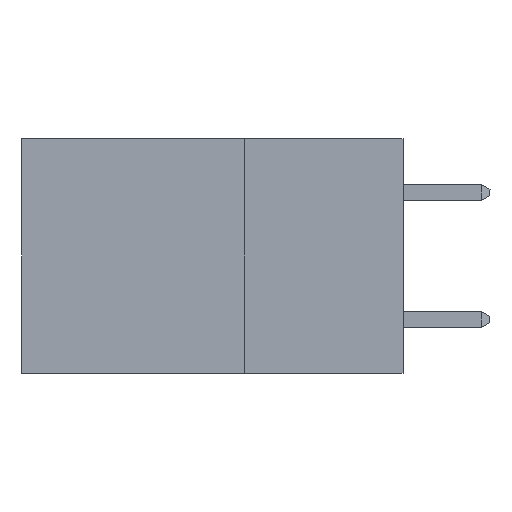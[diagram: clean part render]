
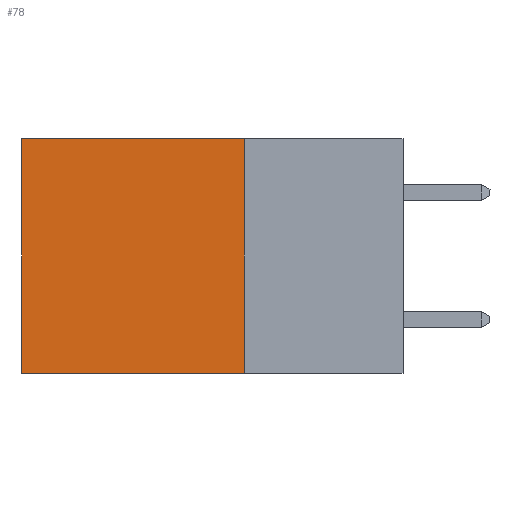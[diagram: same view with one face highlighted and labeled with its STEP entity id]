
A CAD part, left-side view. The second image highlights one B-rep face of the part: STEP entity #78.
In plain terms, the highlighted planar face has unit normal (-1, 0, 0).
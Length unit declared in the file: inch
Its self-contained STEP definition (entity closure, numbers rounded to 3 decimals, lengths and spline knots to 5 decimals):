
#54 = CARTESIAN_POINT ( 'NONE',  ( 0.2875, 0.25, 0. ) ) ;
#78 = ADVANCED_FACE ( 'NONE', ( #9329 ), #5982, .F. ) ;
#121 = DIRECTION ( 'NONE',  ( 0., 0., -1. ) ) ;
#945 = EDGE_CURVE ( 'NONE', #6502, #9573, #3906, .T. ) ;
#1660 = VERTEX_POINT ( 'NONE', #6087 ) ;
#1894 = DIRECTION ( 'NONE',  ( 0., 0., -1. ) ) ;
#2031 = CARTESIAN_POINT ( 'NONE',  ( 0.2875, 0.25, 0. ) ) ;
#2287 = EDGE_CURVE ( 'NONE', #6502, #1660, #8548, .T. ) ;
#2436 = DIRECTION ( 'NONE',  ( 1., 0., 0. ) ) ;
#2835 = DIRECTION ( 'NONE',  ( 0., 1., 0. ) ) ;
#3402 = VECTOR ( 'NONE', #2835, 39.37008 ) ;
#3815 = EDGE_LOOP ( 'NONE', ( #8199, #8211, #8220, #8231 ) ) ;
#3906 = LINE ( 'NONE', #9675, #6200 ) ;
#4716 = CARTESIAN_POINT ( 'NONE',  ( 0.2875, 0.25, -0.37 ) ) ;
#4860 = EDGE_CURVE ( 'NONE', #1660, #6372, #6395, .T. ) ;
#5327 = DIRECTION ( 'NONE',  ( 0., 0., -1. ) ) ;
#5472 = CARTESIAN_POINT ( 'NONE',  ( 0.2875, 0.6, 0. ) ) ;
#5982 = PLANE ( 'NONE',  #8349 ) ;
#6087 = CARTESIAN_POINT ( 'NONE',  ( 0.2875, 0.6, 0. ) ) ;
#6200 = VECTOR ( 'NONE', #1894, 39.37008 ) ;
#6372 = VERTEX_POINT ( 'NONE', #8498 ) ;
#6395 = LINE ( 'NONE', #5472, #10602 ) ;
#6502 = VERTEX_POINT ( 'NONE', #54 ) ;
#7931 = CARTESIAN_POINT ( 'NONE',  ( 0.2875, 0.25, -0.37 ) ) ;
#8134 = CARTESIAN_POINT ( 'NONE',  ( 0.2875, 0.25, 0. ) ) ;
#8199 = ORIENTED_EDGE ( 'NONE', *, *, #4860, .T. ) ;
#8211 = ORIENTED_EDGE ( 'NONE', *, *, #8824, .F. ) ;
#8220 = ORIENTED_EDGE ( 'NONE', *, *, #945, .F. ) ;
#8231 = ORIENTED_EDGE ( 'NONE', *, *, #2287, .T. ) ;
#8349 = AXIS2_PLACEMENT_3D ( 'NONE', #2031, #2436, #121 ) ;
#8498 = CARTESIAN_POINT ( 'NONE',  ( 0.2875, 0.6, -0.37 ) ) ;
#8548 = LINE ( 'NONE', #8134, #10646 ) ;
#8718 = DIRECTION ( 'NONE',  ( 0., 1., 0. ) ) ;
#8824 = EDGE_CURVE ( 'NONE', #9573, #6372, #10001, .T. ) ;
#9329 = FACE_OUTER_BOUND ( 'NONE', #3815, .T. ) ;
#9573 = VERTEX_POINT ( 'NONE', #4716 ) ;
#9675 = CARTESIAN_POINT ( 'NONE',  ( 0.2875, 0.25, 0. ) ) ;
#10001 = LINE ( 'NONE', #7931, #3402 ) ;
#10602 = VECTOR ( 'NONE', #5327, 39.37008 ) ;
#10646 = VECTOR ( 'NONE', #8718, 39.37008 ) ;
